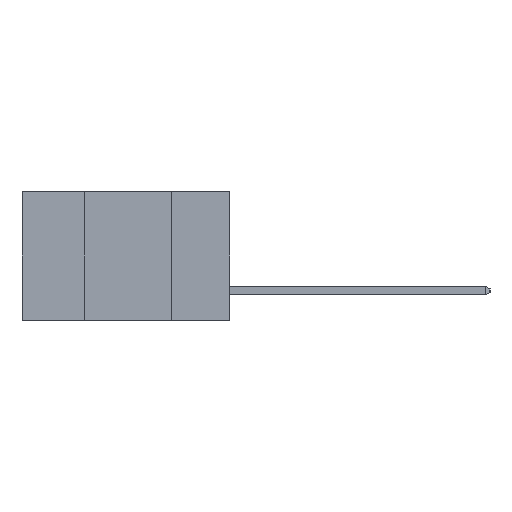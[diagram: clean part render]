
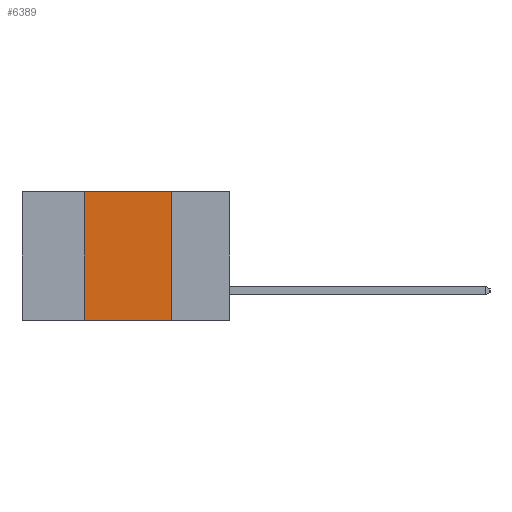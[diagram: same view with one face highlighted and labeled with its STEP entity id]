
A CAD part, left-side view. The second image highlights one B-rep face of the part: STEP entity #6389.
In plain terms, the highlighted planar face has unit normal (-1, 0, 0).
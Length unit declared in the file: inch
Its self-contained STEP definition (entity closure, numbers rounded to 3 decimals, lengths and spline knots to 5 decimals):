
#128 = DIRECTION ( 'NONE',  ( 1., 0., 0. ) ) ;
#768 = VECTOR ( 'NONE', #3251, 39.37008 ) ;
#773 = ORIENTED_EDGE ( 'NONE', *, *, #4475, .F. ) ;
#823 = ORIENTED_EDGE ( 'NONE', *, *, #3627, .F. ) ;
#882 = ORIENTED_EDGE ( 'NONE', *, *, #2793, .F. ) ;
#1019 = ORIENTED_EDGE ( 'NONE', *, *, #1932, .T. ) ;
#1150 = DIRECTION ( 'NONE',  ( 0., -1., 0. ) ) ;
#1206 = LINE ( 'NONE', #6595, #4160 ) ;
#1257 = CARTESIAN_POINT ( 'NONE',  ( 0., 0.17, -0.37 ) ) ;
#1914 = VECTOR ( 'NONE', #1150, 39.37008 ) ;
#1932 = EDGE_CURVE ( 'NONE', #6417, #4698, #1206, .T. ) ;
#2295 = AXIS2_PLACEMENT_3D ( 'NONE', #7755, #128, #8992 ) ;
#2744 = CARTESIAN_POINT ( 'NONE',  ( 0., 0.42, -0.37 ) ) ;
#2793 = EDGE_CURVE ( 'NONE', #6417, #8489, #4129, .T. ) ;
#3251 = DIRECTION ( 'NONE',  ( 0., 0., 1. ) ) ;
#3627 = EDGE_CURVE ( 'NONE', #8489, #3717, #14453, .T. ) ;
#3717 = VERTEX_POINT ( 'NONE', #6272 ) ;
#4129 = LINE ( 'NONE', #5187, #768 ) ;
#4160 = VECTOR ( 'NONE', #6885, 39.37008 ) ;
#4475 = EDGE_CURVE ( 'NONE', #3717, #4698, #13685, .T. ) ;
#4698 = VERTEX_POINT ( 'NONE', #1257 ) ;
#5187 = CARTESIAN_POINT ( 'NONE',  ( 0., 0.42, -0.37 ) ) ;
#6272 = CARTESIAN_POINT ( 'NONE',  ( 0., 0.17, 0. ) ) ;
#6389 = ADVANCED_FACE ( 'NONE', ( #7197 ), #12717, .F. ) ;
#6417 = VERTEX_POINT ( 'NONE', #2744 ) ;
#6595 = CARTESIAN_POINT ( 'NONE',  ( 0., 0.6, -0.37 ) ) ;
#6885 = DIRECTION ( 'NONE',  ( 0., -1., 0. ) ) ;
#6954 = CARTESIAN_POINT ( 'NONE',  ( 0., 0.17, -0.37 ) ) ;
#7068 = VECTOR ( 'NONE', #7457, 39.37008 ) ;
#7197 = FACE_OUTER_BOUND ( 'NONE', #11944, .T. ) ;
#7457 = DIRECTION ( 'NONE',  ( 0., 0., -1. ) ) ;
#7755 = CARTESIAN_POINT ( 'NONE',  ( 0., 0.6, 0. ) ) ;
#8489 = VERTEX_POINT ( 'NONE', #10821 ) ;
#8992 = DIRECTION ( 'NONE',  ( 0., 0., -1. ) ) ;
#10821 = CARTESIAN_POINT ( 'NONE',  ( 0., 0.42, 0. ) ) ;
#11944 = EDGE_LOOP ( 'NONE', ( #773, #823, #882, #1019 ) ) ;
#12674 = CARTESIAN_POINT ( 'NONE',  ( 0., 0.6, 0. ) ) ;
#12717 = PLANE ( 'NONE',  #2295 ) ;
#13685 = LINE ( 'NONE', #6954, #7068 ) ;
#14453 = LINE ( 'NONE', #12674, #1914 ) ;
